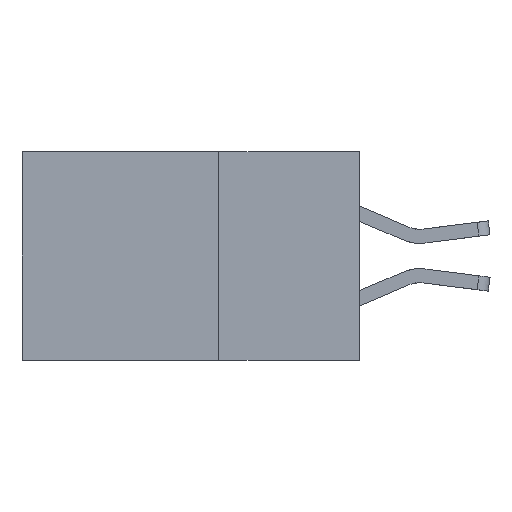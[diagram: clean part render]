
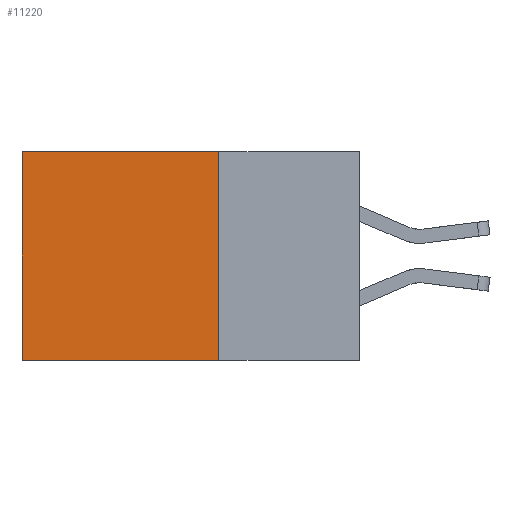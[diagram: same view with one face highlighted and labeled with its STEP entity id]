
A CAD part, left-side view. The second image highlights one B-rep face of the part: STEP entity #11220.
In plain terms, the highlighted planar face has unit normal (-1, 0, 0).
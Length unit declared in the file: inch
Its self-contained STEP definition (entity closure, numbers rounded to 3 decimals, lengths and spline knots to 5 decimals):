
#235 = VERTEX_POINT ( 'NONE', #1742 ) ;
#401 = LINE ( 'NONE', #3607, #1665 ) ;
#546 = EDGE_CURVE ( 'NONE', #235, #8648, #401, .T. ) ;
#732 = CARTESIAN_POINT ( 'NONE',  ( 0.2875, 0.6, -0.37 ) ) ;
#1281 = VERTEX_POINT ( 'NONE', #8499 ) ;
#1665 = VECTOR ( 'NONE', #9096, 39.37008 ) ;
#1742 = CARTESIAN_POINT ( 'NONE',  ( 0.2875, 0.6, 0. ) ) ;
#2210 = CARTESIAN_POINT ( 'NONE',  ( 0.2875, 0.25, 0. ) ) ;
#2330 = CARTESIAN_POINT ( 'NONE',  ( 0.2875, 0.25, -0.37 ) ) ;
#2664 = AXIS2_PLACEMENT_3D ( 'NONE', #10250, #9324, #4760 ) ;
#3471 = LINE ( 'NONE', #11036, #3624 ) ;
#3607 = CARTESIAN_POINT ( 'NONE',  ( 0.2875, 0.6, 0. ) ) ;
#3624 = VECTOR ( 'NONE', #3974, 39.37008 ) ;
#3974 = DIRECTION ( 'NONE',  ( 0., 1., 0. ) ) ;
#4645 = PLANE ( 'NONE',  #2664 ) ;
#4740 = ORIENTED_EDGE ( 'NONE', *, *, #546, .T. ) ;
#4760 = DIRECTION ( 'NONE',  ( 0., 0., -1. ) ) ;
#4967 = CARTESIAN_POINT ( 'NONE',  ( 0.2875, 0.25, 0. ) ) ;
#5105 = EDGE_CURVE ( 'NONE', #1281, #235, #7139, .T. ) ;
#5451 = ORIENTED_EDGE ( 'NONE', *, *, #9159, .F. ) ;
#5564 = ORIENTED_EDGE ( 'NONE', *, *, #5105, .T. ) ;
#6183 = EDGE_LOOP ( 'NONE', ( #4740, #11830, #5451, #5564 ) ) ;
#6535 = DIRECTION ( 'NONE',  ( 0., 1., 0. ) ) ;
#6727 = FACE_OUTER_BOUND ( 'NONE', #6183, .T. ) ;
#6752 = VERTEX_POINT ( 'NONE', #2330 ) ;
#7139 = LINE ( 'NONE', #2210, #11766 ) ;
#8499 = CARTESIAN_POINT ( 'NONE',  ( 0.2875, 0.25, 0. ) ) ;
#8634 = VECTOR ( 'NONE', #11674, 39.37008 ) ;
#8648 = VERTEX_POINT ( 'NONE', #732 ) ;
#9096 = DIRECTION ( 'NONE',  ( 0., 0., -1. ) ) ;
#9159 = EDGE_CURVE ( 'NONE', #1281, #6752, #9220, .T. ) ;
#9220 = LINE ( 'NONE', #4967, #8634 ) ;
#9324 = DIRECTION ( 'NONE',  ( 1., 0., 0. ) ) ;
#9376 = EDGE_CURVE ( 'NONE', #6752, #8648, #3471, .T. ) ;
#10250 = CARTESIAN_POINT ( 'NONE',  ( 0.2875, 0.25, 0. ) ) ;
#11036 = CARTESIAN_POINT ( 'NONE',  ( 0.2875, 0.25, -0.37 ) ) ;
#11220 = ADVANCED_FACE ( 'NONE', ( #6727 ), #4645, .F. ) ;
#11674 = DIRECTION ( 'NONE',  ( 0., 0., -1. ) ) ;
#11766 = VECTOR ( 'NONE', #6535, 39.37008 ) ;
#11830 = ORIENTED_EDGE ( 'NONE', *, *, #9376, .F. ) ;
